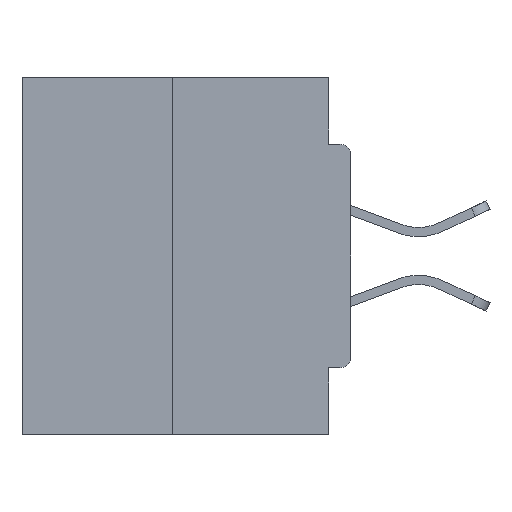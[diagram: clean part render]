
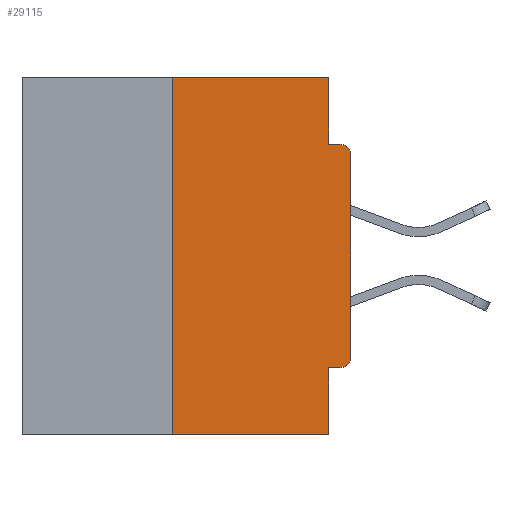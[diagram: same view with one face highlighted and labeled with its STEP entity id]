
A CAD part, left-side view. The second image highlights one B-rep face of the part: STEP entity #29115.
In plain terms, the highlighted planar face has unit normal (-1, 0, 0).
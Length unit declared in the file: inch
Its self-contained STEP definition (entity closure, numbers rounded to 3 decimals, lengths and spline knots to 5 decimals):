
#595 = FACE_OUTER_BOUND ( 'NONE', #27411, .T. ) ;
#783 = ORIENTED_EDGE ( 'NONE', *, *, #2797, .F. ) ;
#1794 = CARTESIAN_POINT ( 'NONE',  ( 0., 0.25, 0. ) ) ;
#2017 = VECTOR ( 'NONE', #23218, 39.37008 ) ;
#2120 = EDGE_CURVE ( 'NONE', #35368, #10610, #6130, .T. ) ;
#2353 = EDGE_CURVE ( 'NONE', #10238, #11780, #7458, .T. ) ;
#2448 = CARTESIAN_POINT ( 'NONE',  ( 0., 0., -0.0935 ) ) ;
#2797 = EDGE_CURVE ( 'NONE', #33920, #11780, #20469, .T. ) ;
#3017 = ORIENTED_EDGE ( 'NONE', *, *, #29820, .T. ) ;
#4275 = CARTESIAN_POINT ( 'NONE',  ( 0., 0.015, -0.4065 ) ) ;
#4450 = CIRCLE ( 'NONE', #34453, 0.015 ) ;
#4629 = ORIENTED_EDGE ( 'NONE', *, *, #31824, .T. ) ;
#6051 = EDGE_CURVE ( 'NONE', #21290, #33920, #12175, .T. ) ;
#6130 = LINE ( 'NONE', #2448, #24583 ) ;
#6679 = CARTESIAN_POINT ( 'NONE',  ( 0., 0., 0. ) ) ;
#6735 = EDGE_CURVE ( 'NONE', #16001, #10610, #4450, .T. ) ;
#7442 = VERTEX_POINT ( 'NONE', #11040 ) ;
#7458 = LINE ( 'NONE', #18420, #25045 ) ;
#7629 = PLANE ( 'NONE',  #8271 ) ;
#7691 = DIRECTION ( 'NONE',  ( 0., 0., -1. ) ) ;
#7925 = CARTESIAN_POINT ( 'NONE',  ( 0., 0.031, -0.4065 ) ) ;
#8271 = AXIS2_PLACEMENT_3D ( 'NONE', #36359, #16961, #22902 ) ;
#8350 = CARTESIAN_POINT ( 'NONE',  ( 0., 0.25, 0. ) ) ;
#8408 = ORIENTED_EDGE ( 'NONE', *, *, #2353, .T. ) ;
#9222 = DIRECTION ( 'NONE',  ( 0., 0., -1. ) ) ;
#9384 = ORIENTED_EDGE ( 'NONE', *, *, #36813, .F. ) ;
#9629 = ORIENTED_EDGE ( 'NONE', *, *, #6735, .T. ) ;
#10238 = VERTEX_POINT ( 'NONE', #28427 ) ;
#10610 = VERTEX_POINT ( 'NONE', #29397 ) ;
#11040 = CARTESIAN_POINT ( 'NONE',  ( 0., 0.031, 0. ) ) ;
#11418 = ORIENTED_EDGE ( 'NONE', *, *, #25586, .F. ) ;
#11780 = VERTEX_POINT ( 'NONE', #27265 ) ;
#11819 = ORIENTED_EDGE ( 'NONE', *, *, #32379, .F. ) ;
#11920 = DIRECTION ( 'NONE',  ( 0., 1., 0. ) ) ;
#12175 = LINE ( 'NONE', #29283, #25662 ) ;
#12515 = DIRECTION ( 'NONE',  ( 0., -1., 0. ) ) ;
#13113 = VECTOR ( 'NONE', #9222, 39.37008 ) ;
#13585 = ORIENTED_EDGE ( 'NONE', *, *, #2120, .F. ) ;
#13885 = VECTOR ( 'NONE', #22852, 39.37008 ) ;
#14464 = VECTOR ( 'NONE', #35786, 39.37008 ) ;
#15162 = DIRECTION ( 'NONE',  ( 0., -1., 0. ) ) ;
#15362 = LINE ( 'NONE', #6679, #14464 ) ;
#15486 = CARTESIAN_POINT ( 'NONE',  ( 0., 0.031, 0. ) ) ;
#16001 = VERTEX_POINT ( 'NONE', #26313 ) ;
#16764 = CARTESIAN_POINT ( 'NONE',  ( 0., 0.015, -0.1085 ) ) ;
#16961 = DIRECTION ( 'NONE',  ( 1., 0., 0. ) ) ;
#18420 = CARTESIAN_POINT ( 'NONE',  ( 0., 0.46, -0.5 ) ) ;
#18702 = VERTEX_POINT ( 'NONE', #1794 ) ;
#19175 = DIRECTION ( 'NONE',  ( -1., 0., 0. ) ) ;
#20469 = LINE ( 'NONE', #35051, #2017 ) ;
#21290 = VERTEX_POINT ( 'NONE', #4275 ) ;
#22471 = LINE ( 'NONE', #8350, #13885 ) ;
#22852 = DIRECTION ( 'NONE',  ( 0., 0., 1. ) ) ;
#22870 = ORIENTED_EDGE ( 'NONE', *, *, #6051, .F. ) ;
#22902 = DIRECTION ( 'NONE',  ( 0., 0., -1. ) ) ;
#23056 = LINE ( 'NONE', #15486, #13113 ) ;
#23218 = DIRECTION ( 'NONE',  ( 0., 0., -1. ) ) ;
#24583 = VECTOR ( 'NONE', #34933, 39.37008 ) ;
#25045 = VECTOR ( 'NONE', #12515, 39.37008 ) ;
#25203 = LINE ( 'NONE', #26356, #27912 ) ;
#25586 = EDGE_CURVE ( 'NONE', #18702, #7442, #25203, .T. ) ;
#25662 = VECTOR ( 'NONE', #11920, 39.37008 ) ;
#25748 = DIRECTION ( 'NONE',  ( -1., 0., 0. ) ) ;
#26313 = CARTESIAN_POINT ( 'NONE',  ( 0., 0., -0.1085 ) ) ;
#26356 = CARTESIAN_POINT ( 'NONE',  ( 0., 0.46, 0. ) ) ;
#27265 = CARTESIAN_POINT ( 'NONE',  ( 0., 0.031, -0.5 ) ) ;
#27411 = EDGE_LOOP ( 'NONE', ( #11418, #11819, #8408, #783, #22870, #4629, #3017, #9629, #13585, #9384 ) ) ;
#27855 = CARTESIAN_POINT ( 'NONE',  ( 0., 0., -0.3915 ) ) ;
#27912 = VECTOR ( 'NONE', #15162, 39.37008 ) ;
#28427 = CARTESIAN_POINT ( 'NONE',  ( 0., 0.25, -0.5 ) ) ;
#28520 = CARTESIAN_POINT ( 'NONE',  ( 0., 0.015, -0.3915 ) ) ;
#29115 = ADVANCED_FACE ( 'NONE', ( #595 ), #7629, .F. ) ;
#29283 = CARTESIAN_POINT ( 'NONE',  ( 0., 0., -0.4065 ) ) ;
#29397 = CARTESIAN_POINT ( 'NONE',  ( 0., 0.015, -0.0935 ) ) ;
#29728 = CIRCLE ( 'NONE', #30063, 0.015 ) ;
#29820 = EDGE_CURVE ( 'NONE', #31274, #16001, #15362, .T. ) ;
#30063 = AXIS2_PLACEMENT_3D ( 'NONE', #28520, #25748, #31429 ) ;
#31274 = VERTEX_POINT ( 'NONE', #27855 ) ;
#31429 = DIRECTION ( 'NONE',  ( 0., 0., -1. ) ) ;
#31493 = CARTESIAN_POINT ( 'NONE',  ( 0., 0.031, -0.0935 ) ) ;
#31824 = EDGE_CURVE ( 'NONE', #21290, #31274, #29728, .T. ) ;
#32379 = EDGE_CURVE ( 'NONE', #10238, #18702, #22471, .T. ) ;
#33920 = VERTEX_POINT ( 'NONE', #7925 ) ;
#34453 = AXIS2_PLACEMENT_3D ( 'NONE', #16764, #19175, #7691 ) ;
#34933 = DIRECTION ( 'NONE',  ( 0., -1., 0. ) ) ;
#35051 = CARTESIAN_POINT ( 'NONE',  ( 0., 0.031, -0.5 ) ) ;
#35368 = VERTEX_POINT ( 'NONE', #31493 ) ;
#35786 = DIRECTION ( 'NONE',  ( 0., 0., 1. ) ) ;
#36359 = CARTESIAN_POINT ( 'NONE',  ( 0., 0.46, 0. ) ) ;
#36813 = EDGE_CURVE ( 'NONE', #7442, #35368, #23056, .T. ) ;
